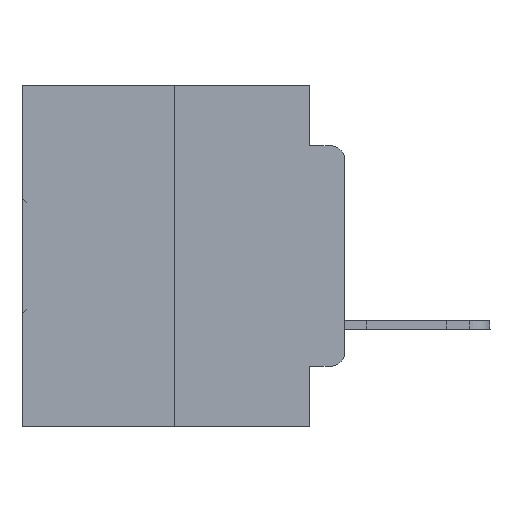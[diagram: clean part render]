
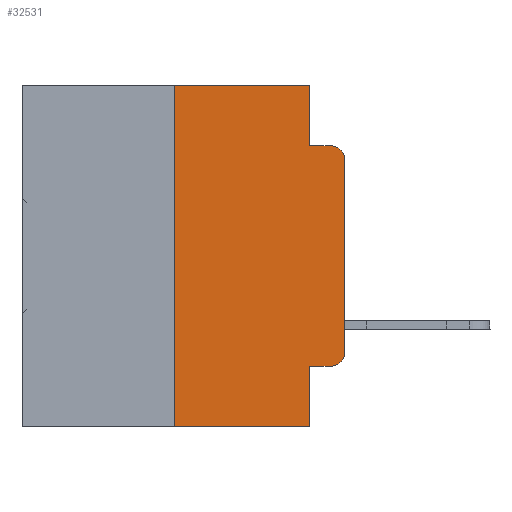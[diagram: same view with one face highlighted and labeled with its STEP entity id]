
A CAD part, left-side view. The second image highlights one B-rep face of the part: STEP entity #32531.
In plain terms, the highlighted planar face has unit normal (-1, 0, 0).
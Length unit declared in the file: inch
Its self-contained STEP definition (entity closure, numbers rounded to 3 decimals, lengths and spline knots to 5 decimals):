
#279 = DIRECTION ( 'NONE',  ( 0., -1., 0. ) ) ;
#800 = DIRECTION ( 'NONE',  ( 0., 0., -1. ) ) ;
#981 = DIRECTION ( 'NONE',  ( -1., 0., 0. ) ) ;
#1615 = VERTEX_POINT ( 'NONE', #2531 ) ;
#1853 = CARTESIAN_POINT ( 'NONE',  ( 0., 0.02, -0.3915 ) ) ;
#2513 = CARTESIAN_POINT ( 'NONE',  ( 0., 0.473, 0. ) ) ;
#2531 = CARTESIAN_POINT ( 'NONE',  ( 0., 0.051, 0. ) ) ;
#2668 = VECTOR ( 'NONE', #6933, 39.37008 ) ;
#3119 = ORIENTED_EDGE ( 'NONE', *, *, #25107, .T. ) ;
#3386 = EDGE_CURVE ( 'NONE', #17190, #28097, #17893, .T. ) ;
#3653 = DIRECTION ( 'NONE',  ( 0., 0., -1. ) ) ;
#3959 = CARTESIAN_POINT ( 'NONE',  ( 0., 0.25, 0. ) ) ;
#4526 = DIRECTION ( 'NONE',  ( -1., 0., 0. ) ) ;
#5196 = VERTEX_POINT ( 'NONE', #32049 ) ;
#5919 = CARTESIAN_POINT ( 'NONE',  ( 0., 0.051, -0.0885 ) ) ;
#6163 = EDGE_LOOP ( 'NONE', ( #10452, #26785, #27700, #28177, #19234, #29250, #3119, #25181, #20458, #11862 ) ) ;
#6933 = DIRECTION ( 'NONE',  ( 0., 0., 1. ) ) ;
#9618 = LINE ( 'NONE', #24040, #32396 ) ;
#9739 = EDGE_CURVE ( 'NONE', #5196, #22600, #17716, .T. ) ;
#9841 = EDGE_CURVE ( 'NONE', #22600, #33943, #31809, .T. ) ;
#10452 = ORIENTED_EDGE ( 'NONE', *, *, #9739, .T. ) ;
#11061 = EDGE_CURVE ( 'NONE', #1615, #14852, #26326, .T. ) ;
#11516 = VECTOR ( 'NONE', #29755, 39.37008 ) ;
#11524 = VECTOR ( 'NONE', #20636, 39.37008 ) ;
#11862 = ORIENTED_EDGE ( 'NONE', *, *, #31857, .T. ) ;
#12204 = CARTESIAN_POINT ( 'NONE',  ( 0., 0.473, -0.5 ) ) ;
#12636 = LINE ( 'NONE', #17915, #2668 ) ;
#12664 = VECTOR ( 'NONE', #800, 39.37008 ) ;
#12697 = DIRECTION ( 'NONE',  ( 0., -1., 0. ) ) ;
#13383 = VERTEX_POINT ( 'NONE', #19993 ) ;
#14014 = LINE ( 'NONE', #16479, #11516 ) ;
#14344 = EDGE_CURVE ( 'NONE', #17677, #1615, #9618, .T. ) ;
#14399 = VECTOR ( 'NONE', #12697, 39.37008 ) ;
#14852 = VERTEX_POINT ( 'NONE', #5919 ) ;
#15356 = CARTESIAN_POINT ( 'NONE',  ( 0., 0.02, -0.4115 ) ) ;
#15376 = CARTESIAN_POINT ( 'NONE',  ( 0., 0., -0.1085 ) ) ;
#15437 = DIRECTION ( 'NONE',  ( 0., -1., 0. ) ) ;
#16479 = CARTESIAN_POINT ( 'NONE',  ( 0., 0.051, 0. ) ) ;
#16772 = AXIS2_PLACEMENT_3D ( 'NONE', #1853, #4526, #28948 ) ;
#16917 = CARTESIAN_POINT ( 'NONE',  ( 0., 0.051, 0. ) ) ;
#16974 = CARTESIAN_POINT ( 'NONE',  ( 0., 0.051, -0.5 ) ) ;
#17190 = VERTEX_POINT ( 'NONE', #30859 ) ;
#17219 = AXIS2_PLACEMENT_3D ( 'NONE', #2513, #28420, #23837 ) ;
#17677 = VERTEX_POINT ( 'NONE', #3959 ) ;
#17716 = LINE ( 'NONE', #28061, #11524 ) ;
#17893 = LINE ( 'NONE', #25802, #19920 ) ;
#17915 = CARTESIAN_POINT ( 'NONE',  ( 0., 0.25, 0. ) ) ;
#19234 = ORIENTED_EDGE ( 'NONE', *, *, #14344, .F. ) ;
#19844 = CARTESIAN_POINT ( 'NONE',  ( 0., 0.02, -0.1085 ) ) ;
#19920 = VECTOR ( 'NONE', #15437, 39.37008 ) ;
#19993 = CARTESIAN_POINT ( 'NONE',  ( 0., 0.25, -0.5 ) ) ;
#20458 = ORIENTED_EDGE ( 'NONE', *, *, #3386, .T. ) ;
#20483 = EDGE_CURVE ( 'NONE', #14852, #33943, #20568, .T. ) ;
#20568 = LINE ( 'NONE', #23451, #14399 ) ;
#20636 = DIRECTION ( 'NONE',  ( 0., 0., 1. ) ) ;
#21716 = CARTESIAN_POINT ( 'NONE',  ( 0., 0.02, -0.0885 ) ) ;
#21812 = AXIS2_PLACEMENT_3D ( 'NONE', #19844, #981, #3653 ) ;
#21908 = EDGE_CURVE ( 'NONE', #13383, #17677, #12636, .T. ) ;
#22600 = VERTEX_POINT ( 'NONE', #15376 ) ;
#23451 = CARTESIAN_POINT ( 'NONE',  ( 0., 0.051, -0.0885 ) ) ;
#23837 = DIRECTION ( 'NONE',  ( 0., 0., -1. ) ) ;
#24040 = CARTESIAN_POINT ( 'NONE',  ( 0., 0.473, 0. ) ) ;
#25107 = EDGE_CURVE ( 'NONE', #13383, #34096, #30695, .T. ) ;
#25180 = CIRCLE ( 'NONE', #16772, 0.02 ) ;
#25181 = ORIENTED_EDGE ( 'NONE', *, *, #27280, .F. ) ;
#25295 = VECTOR ( 'NONE', #33579, 39.37008 ) ;
#25544 = FACE_OUTER_BOUND ( 'NONE', #6163, .T. ) ;
#25802 = CARTESIAN_POINT ( 'NONE',  ( 0., 0.051, -0.4115 ) ) ;
#26326 = LINE ( 'NONE', #16917, #12664 ) ;
#26785 = ORIENTED_EDGE ( 'NONE', *, *, #9841, .T. ) ;
#27280 = EDGE_CURVE ( 'NONE', #17190, #34096, #14014, .T. ) ;
#27700 = ORIENTED_EDGE ( 'NONE', *, *, #20483, .F. ) ;
#28061 = CARTESIAN_POINT ( 'NONE',  ( 0., 0., 0. ) ) ;
#28097 = VERTEX_POINT ( 'NONE', #15356 ) ;
#28177 = ORIENTED_EDGE ( 'NONE', *, *, #11061, .F. ) ;
#28420 = DIRECTION ( 'NONE',  ( 1., 0., 0. ) ) ;
#28948 = DIRECTION ( 'NONE',  ( 0., 0., -1. ) ) ;
#29250 = ORIENTED_EDGE ( 'NONE', *, *, #21908, .F. ) ;
#29755 = DIRECTION ( 'NONE',  ( 0., 0., -1. ) ) ;
#30695 = LINE ( 'NONE', #12204, #25295 ) ;
#30859 = CARTESIAN_POINT ( 'NONE',  ( 0., 0.051, -0.4115 ) ) ;
#31809 = CIRCLE ( 'NONE', #21812, 0.02 ) ;
#31857 = EDGE_CURVE ( 'NONE', #28097, #5196, #25180, .T. ) ;
#32049 = CARTESIAN_POINT ( 'NONE',  ( 0., 0., -0.3915 ) ) ;
#32396 = VECTOR ( 'NONE', #279, 39.37008 ) ;
#32531 = ADVANCED_FACE ( 'NONE', ( #25544 ), #34229, .F. ) ;
#33579 = DIRECTION ( 'NONE',  ( 0., -1., 0. ) ) ;
#33943 = VERTEX_POINT ( 'NONE', #21716 ) ;
#34096 = VERTEX_POINT ( 'NONE', #16974 ) ;
#34229 = PLANE ( 'NONE',  #17219 ) ;
